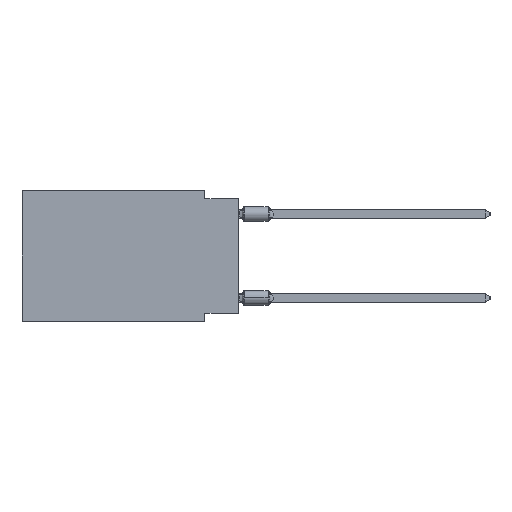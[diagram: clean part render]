
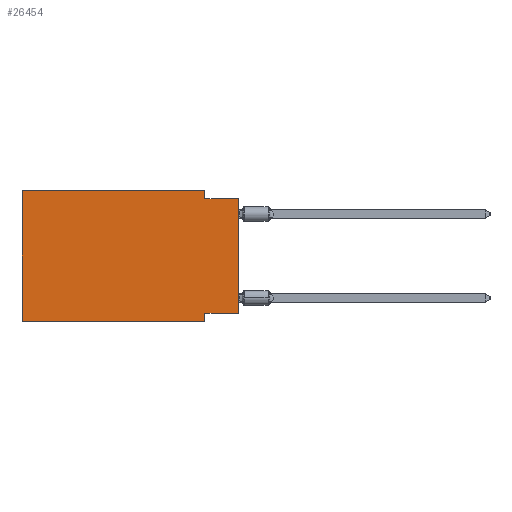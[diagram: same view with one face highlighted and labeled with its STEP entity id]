
A CAD part, left-side view. The second image highlights one B-rep face of the part: STEP entity #26454.
In plain terms, the highlighted planar face has unit normal (-1, 0, 0).
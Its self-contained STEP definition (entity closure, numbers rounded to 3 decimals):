
#221 = VECTOR ( 'NONE', #59688, 1000. ) ;
#341 = DIRECTION ( 'NONE',  ( 0., 1., 0. ) ) ;
#2031 = EDGE_CURVE ( 'NONE', #59616, #47728, #34033, .T. ) ;
#4514 = CARTESIAN_POINT ( 'NONE',  ( 0., 16.383, 0. ) ) ;
#5782 = VECTOR ( 'NONE', #49204, 1000. ) ;
#8218 = CARTESIAN_POINT ( 'NONE',  ( 0., 2.54, -9.271 ) ) ;
#8695 = LINE ( 'NONE', #18981, #221 ) ;
#10784 = VERTEX_POINT ( 'NONE', #13195 ) ;
#12399 = CARTESIAN_POINT ( 'NONE',  ( 0., 0., -0.635 ) ) ;
#13160 = DIRECTION ( 'NONE',  ( 0., 0., -1. ) ) ;
#13195 = CARTESIAN_POINT ( 'NONE',  ( 0., 0., -0.635 ) ) ;
#14281 = EDGE_CURVE ( 'NONE', #38555, #10784, #39075, .T. ) ;
#14509 = VERTEX_POINT ( 'NONE', #35958 ) ;
#16685 = EDGE_CURVE ( 'NONE', #64860, #42867, #65067, .T. ) ;
#17175 = DIRECTION ( 'NONE',  ( 0., -1., 0. ) ) ;
#17568 = EDGE_CURVE ( 'NONE', #29562, #38555, #33351, .T. ) ;
#18196 = LINE ( 'NONE', #63706, #25507 ) ;
#18981 = CARTESIAN_POINT ( 'NONE',  ( 0., 16.383, -9.906 ) ) ;
#19874 = EDGE_LOOP ( 'NONE', ( #55755, #58187, #45413, #29067, #27311, #25532, #33000, #61283 ) ) ;
#23229 = LINE ( 'NONE', #65978, #5782 ) ;
#25507 = VECTOR ( 'NONE', #17175, 1000. ) ;
#25532 = ORIENTED_EDGE ( 'NONE', *, *, #30287, .T. ) ;
#26454 = ADVANCED_FACE ( 'NONE', ( #27174 ), #37776, .F. ) ;
#27112 = CARTESIAN_POINT ( 'NONE',  ( 0., 2.54, -9.906 ) ) ;
#27174 = FACE_OUTER_BOUND ( 'NONE', #19874, .T. ) ;
#27311 = ORIENTED_EDGE ( 'NONE', *, *, #2031, .F. ) ;
#27454 = DIRECTION ( 'NONE',  ( 0., -1., 0. ) ) ;
#27682 = VECTOR ( 'NONE', #64827, 1000. ) ;
#29067 = ORIENTED_EDGE ( 'NONE', *, *, #58114, .F. ) ;
#29562 = VERTEX_POINT ( 'NONE', #30798 ) ;
#30287 = EDGE_CURVE ( 'NONE', #59616, #42867, #8695, .T. ) ;
#30399 = VECTOR ( 'NONE', #13160, 1000. ) ;
#30441 = AXIS2_PLACEMENT_3D ( 'NONE', #58972, #53173, #42903 ) ;
#30798 = CARTESIAN_POINT ( 'NONE',  ( 0., 2.54, 0. ) ) ;
#33000 = ORIENTED_EDGE ( 'NONE', *, *, #16685, .F. ) ;
#33351 = LINE ( 'NONE', #60025, #30399 ) ;
#34033 = LINE ( 'NONE', #53879, #27682 ) ;
#35958 = CARTESIAN_POINT ( 'NONE',  ( 0., 0., -9.271 ) ) ;
#36109 = EDGE_CURVE ( 'NONE', #14509, #64860, #58145, .T. ) ;
#37776 = PLANE ( 'NONE',  #30441 ) ;
#38555 = VERTEX_POINT ( 'NONE', #62950 ) ;
#39075 = LINE ( 'NONE', #12399, #67437 ) ;
#41339 = CARTESIAN_POINT ( 'NONE',  ( 0., 16.383, -9.906 ) ) ;
#42066 = CARTESIAN_POINT ( 'NONE',  ( 0., 0., -9.271 ) ) ;
#42867 = VERTEX_POINT ( 'NONE', #52882 ) ;
#42903 = DIRECTION ( 'NONE',  ( 0., 0., -1. ) ) ;
#43506 = DIRECTION ( 'NONE',  ( 0., 0., -1. ) ) ;
#45413 = ORIENTED_EDGE ( 'NONE', *, *, #17568, .F. ) ;
#45532 = VECTOR ( 'NONE', #341, 1000. ) ;
#47728 = VERTEX_POINT ( 'NONE', #4514 ) ;
#49204 = DIRECTION ( 'NONE',  ( 0., 0., 1. ) ) ;
#49597 = EDGE_CURVE ( 'NONE', #14509, #10784, #23229, .T. ) ;
#52882 = CARTESIAN_POINT ( 'NONE',  ( 0., 2.54, -9.906 ) ) ;
#53173 = DIRECTION ( 'NONE',  ( 1., 0., 0. ) ) ;
#53879 = CARTESIAN_POINT ( 'NONE',  ( 0., 16.383, 0. ) ) ;
#54341 = VECTOR ( 'NONE', #43506, 1000. ) ;
#55755 = ORIENTED_EDGE ( 'NONE', *, *, #49597, .T. ) ;
#58114 = EDGE_CURVE ( 'NONE', #47728, #29562, #18196, .T. ) ;
#58145 = LINE ( 'NONE', #42066, #45532 ) ;
#58187 = ORIENTED_EDGE ( 'NONE', *, *, #14281, .F. ) ;
#58972 = CARTESIAN_POINT ( 'NONE',  ( 0., 16.383, 0. ) ) ;
#59616 = VERTEX_POINT ( 'NONE', #41339 ) ;
#59688 = DIRECTION ( 'NONE',  ( 0., -1., 0. ) ) ;
#60025 = CARTESIAN_POINT ( 'NONE',  ( 0., 2.54, 0. ) ) ;
#61283 = ORIENTED_EDGE ( 'NONE', *, *, #36109, .F. ) ;
#62950 = CARTESIAN_POINT ( 'NONE',  ( 0., 2.54, -0.635 ) ) ;
#63706 = CARTESIAN_POINT ( 'NONE',  ( 0., 16.383, 0. ) ) ;
#64827 = DIRECTION ( 'NONE',  ( 0., 0., 1. ) ) ;
#64860 = VERTEX_POINT ( 'NONE', #8218 ) ;
#65067 = LINE ( 'NONE', #27112, #54341 ) ;
#65978 = CARTESIAN_POINT ( 'NONE',  ( 0., 0., 0. ) ) ;
#67437 = VECTOR ( 'NONE', #27454, 1000. ) ;
